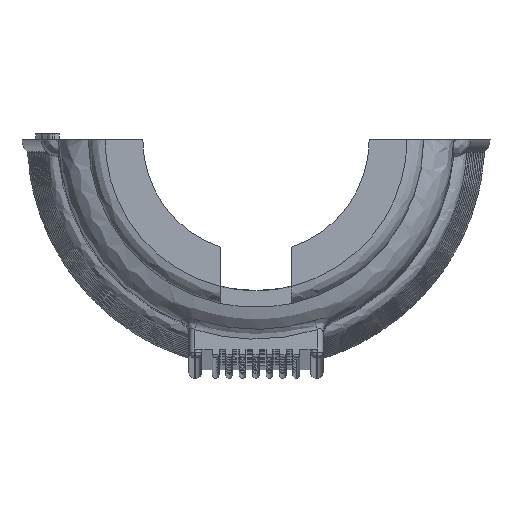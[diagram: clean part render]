
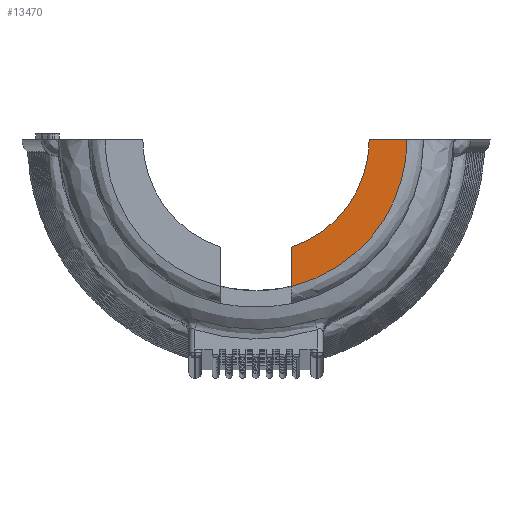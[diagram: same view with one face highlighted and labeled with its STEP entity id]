
A CAD part, left-side view. The second image highlights one B-rep face of the part: STEP entity #13470.
In plain terms, the highlighted planar face has unit normal (-1, 0, 0).
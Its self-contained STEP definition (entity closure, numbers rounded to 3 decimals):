
#179 = CARTESIAN_POINT ( 'NONE',  ( -170., -13.5, 0. ) ) ;
#528 = CARTESIAN_POINT ( 'NONE',  ( -170., -4.2, -17.503 ) ) ;
#675 = CARTESIAN_POINT ( 'NONE',  ( -170., -9.207, -15.468 ) ) ;
#755 = CARTESIAN_POINT ( 'NONE',  ( -170., -13.836, -11.526 ) ) ;
#820 = CARTESIAN_POINT ( 'NONE',  ( -170., -17.05, -5.77 ) ) ;
#1098 = VERTEX_POINT ( 'NONE', #18609 ) ;
#1494 = EDGE_CURVE ( 'NONE', #1098, #16341, #10187, .T. ) ;
#1800 = VERTEX_POINT ( 'NONE', #179 ) ;
#2289 = CARTESIAN_POINT ( 'NONE',  ( -170., -4.2, -17.503 ) ) ;
#2359 = CARTESIAN_POINT ( 'NONE',  ( -170., -9.473, -15.306 ) ) ;
#2428 = CARTESIAN_POINT ( 'NONE',  ( -170., -14.931, -10.077 ) ) ;
#2504 = CARTESIAN_POINT ( 'NONE',  ( -170., -17.434, -4.528 ) ) ;
#3507 = EDGE_LOOP ( 'NONE', ( #18402, #18695, #16686, #12770 ) ) ;
#3976 = CARTESIAN_POINT ( 'NONE',  ( -170., -6.147, -16.921 ) ) ;
#4041 = CARTESIAN_POINT ( 'NONE',  ( -170., -10.014, -14.966 ) ) ;
#4114 = CARTESIAN_POINT ( 'NONE',  ( -170., -15.606, -8.971 ) ) ;
#4183 = CARTESIAN_POINT ( 'NONE',  ( -170., -17.703, -3.259 ) ) ;
#4594 = CARTESIAN_POINT ( 'NONE',  ( -170., 0., 0. ) ) ;
#5428 = EDGE_CURVE ( 'NONE', #1098, #1800, #19788, .T. ) ;
#5637 = CARTESIAN_POINT ( 'NONE',  ( -170., -6.733, -16.694 ) ) ;
#5679 = LINE ( 'NONE', #10400, #14093 ) ;
#5715 = CARTESIAN_POINT ( 'NONE',  ( -170., -11.35, -13.975 ) ) ;
#5782 = CARTESIAN_POINT ( 'NONE',  ( -170., -15.797, -8.63 ) ) ;
#5846 = CARTESIAN_POINT ( 'NONE',  ( -170., -17.756, -2.953 ) ) ;
#6245 = DIRECTION ( 'NONE',  ( 0., 0., 1. ) ) ;
#6304 = DIRECTION ( 'NONE',  ( -1., 0., 0. ) ) ;
#7123 = FACE_OUTER_BOUND ( 'NONE', #3507, .T. ) ;
#7302 = CARTESIAN_POINT ( 'NONE',  ( -170., -6.871, -16.637 ) ) ;
#7372 = CARTESIAN_POINT ( 'NONE',  ( -170., -11.838, -13.56 ) ) ;
#7446 = CARTESIAN_POINT ( 'NONE',  ( -170., -16.432, -7.378 ) ) ;
#7517 = CARTESIAN_POINT ( 'NONE',  ( -170., -17.771, -2.86 ) ) ;
#8326 = EDGE_CURVE ( 'NONE', #16341, #20153, #16764, .T. ) ;
#8989 = CARTESIAN_POINT ( 'NONE',  ( -170., -7.388, -16.422 ) ) ;
#9069 = CARTESIAN_POINT ( 'NONE',  ( -170., -12.417, -13.042 ) ) ;
#9144 = CARTESIAN_POINT ( 'NONE',  ( -170., -16.924, -6.133 ) ) ;
#9216 = CARTESIAN_POINT ( 'NONE',  ( -170., -18., -0.95 ) ) ;
#9973 = AXIS2_PLACEMENT_3D ( 'NONE', #4594, #16332, #6245 ) ;
#10187 = LINE ( 'NONE', #12063, #18598 ) ;
#10400 = CARTESIAN_POINT ( 'NONE',  ( -170., -20.747, 0. ) ) ;
#10544 = CARTESIAN_POINT ( 'NONE',  ( -170., -5.357, -17.196 ) ) ;
#10704 = CARTESIAN_POINT ( 'NONE',  ( -170., -8.83, -15.689 ) ) ;
#10772 = CARTESIAN_POINT ( 'NONE',  ( -170., -13.497, -11.921 ) ) ;
#10846 = CARTESIAN_POINT ( 'NONE',  ( -170., -17.029, -5.832 ) ) ;
#11100 = AXIS2_PLACEMENT_3D ( 'NONE', #21342, #6304, #18062 ) ;
#12063 = CARTESIAN_POINT ( 'NONE',  ( -170., -4.2, -8.804 ) ) ;
#12094 = DIRECTION ( 'NONE',  ( 0., 1., 0. ) ) ;
#12395 = CARTESIAN_POINT ( 'NONE',  ( -170., -9.367, -15.371 ) ) ;
#12473 = CARTESIAN_POINT ( 'NONE',  ( -170., -14.477, -10.709 ) ) ;
#12549 = CARTESIAN_POINT ( 'NONE',  ( -170., -17.227, -5.241 ) ) ;
#12770 = ORIENTED_EDGE ( 'NONE', *, *, #8326, .T. ) ;
#13470 = ADVANCED_FACE ( 'NONE', ( #7123 ), #16390, .T. ) ;
#14088 = CARTESIAN_POINT ( 'NONE',  ( -170., -9.525, -15.274 ) ) ;
#14093 = VECTOR ( 'NONE', #12094, 1000. ) ;
#14164 = CARTESIAN_POINT ( 'NONE',  ( -170., -15.411, -9.308 ) ) ;
#14234 = CARTESIAN_POINT ( 'NONE',  ( -170., -17.622, -3.684 ) ) ;
#15694 = CARTESIAN_POINT ( 'NONE',  ( -170., -6.538, -16.771 ) ) ;
#15763 = CARTESIAN_POINT ( 'NONE',  ( -170., -10.646, -14.53 ) ) ;
#15830 = CARTESIAN_POINT ( 'NONE',  ( -170., -15.733, -8.745 ) ) ;
#15911 = CARTESIAN_POINT ( 'NONE',  ( -170., -17.741, -3.045 ) ) ;
#16055 = CARTESIAN_POINT ( 'NONE',  ( -170., -18., 0. ) ) ;
#16332 = DIRECTION ( 'NONE',  ( -1., 0., 0. ) ) ;
#16341 = VERTEX_POINT ( 'NONE', #528 ) ;
#16390 = PLANE ( 'NONE',  #11100 ) ;
#16686 = ORIENTED_EDGE ( 'NONE', *, *, #1494, .T. ) ;
#16764 = B_SPLINE_CURVE_WITH_KNOTS ( 'NONE', 3,
 ( #2289, #20580, #10544, #3976, #15694, #5637, #17373, #7302, #19057, #8989, #20729, #10704, #675, #12395, #2359, #14088, #4041, #15763, #5715, #17447, #7372, #19127, #9069, #20799, #10772, #755, #12473, #2428, #14164, #4114, #15830, #5782, #17520, #7446, #19190, #9144, #20879, #10846, #820, #12549, #2504, #14234, #4183, #15911, #5846, #17589, #7517, #19267, #9216, #20951 ),
 .UNSPECIFIED., .F., .F.,
 ( 4, 1, 1, 1, 1, 2, 2, 1, 1, 1, 2, 2, 1, 1, 2, 2, 2, 2, 1, 1, 2, 2, 1, 1, 1, 2, 2, 1, 1, 1, 1, 2, 2, 4 ),
 ( 0., 0.062, 0.094, 0.109, 0.117, 0.121, 0.125, 0.187, 0.219, 0.234, 0.242, 0.25, 0.312, 0.344, 0.359, 0.375, 0.437, 0.5, 0.562, 0.594, 0.609, 0.625, 0.687, 0.719, 0.734, 0.742, 0.75, 0.812, 0.844, 0.859, 0.867, 0.871, 0.875, 1. ),
 .UNSPECIFIED. ) ;
#17125 = DIRECTION ( 'NONE',  ( 0., 0., -1. ) ) ;
#17226 = EDGE_CURVE ( 'NONE', #20153, #1800, #5679, .T. ) ;
#17373 = CARTESIAN_POINT ( 'NONE',  ( -170., -6.816, -16.66 ) ) ;
#17447 = CARTESIAN_POINT ( 'NONE',  ( -170., -11.644, -13.727 ) ) ;
#17520 = CARTESIAN_POINT ( 'NONE',  ( -170., -16.099, -8.067 ) ) ;
#17589 = CARTESIAN_POINT ( 'NONE',  ( -170., -17.766, -2.892 ) ) ;
#18062 = DIRECTION ( 'NONE',  ( 0., -1., 0. ) ) ;
#18402 = ORIENTED_EDGE ( 'NONE', *, *, #17226, .T. ) ;
#18598 = VECTOR ( 'NONE', #17125, 1000. ) ;
#18609 = CARTESIAN_POINT ( 'NONE',  ( -170., -4.2, -12.83 ) ) ;
#18695 = ORIENTED_EDGE ( 'NONE', *, *, #5428, .F. ) ;
#19057 = CARTESIAN_POINT ( 'NONE',  ( -170., -6.898, -16.626 ) ) ;
#19127 = CARTESIAN_POINT ( 'NONE',  ( -170., -11.933, -13.476 ) ) ;
#19190 = CARTESIAN_POINT ( 'NONE',  ( -170., -16.769, -6.552 ) ) ;
#19267 = CARTESIAN_POINT ( 'NONE',  ( -170., -17.925, -1.894 ) ) ;
#19788 = CIRCLE ( 'NONE', #9973, 13.5 ) ;
#20153 = VERTEX_POINT ( 'NONE', #16055 ) ;
#20580 = CARTESIAN_POINT ( 'NONE',  ( -170., -4.666, -17.391 ) ) ;
#20729 = CARTESIAN_POINT ( 'NONE',  ( -170., -8.065, -16.106 ) ) ;
#20799 = CARTESIAN_POINT ( 'NONE',  ( -170., -12.788, -12.678 ) ) ;
#20879 = CARTESIAN_POINT ( 'NONE',  ( -170., -16.987, -5.953 ) ) ;
#20951 = CARTESIAN_POINT ( 'NONE',  ( -170., -18., 0. ) ) ;
#21342 = CARTESIAN_POINT ( 'NONE',  ( -170., -4.2, -17.608 ) ) ;
